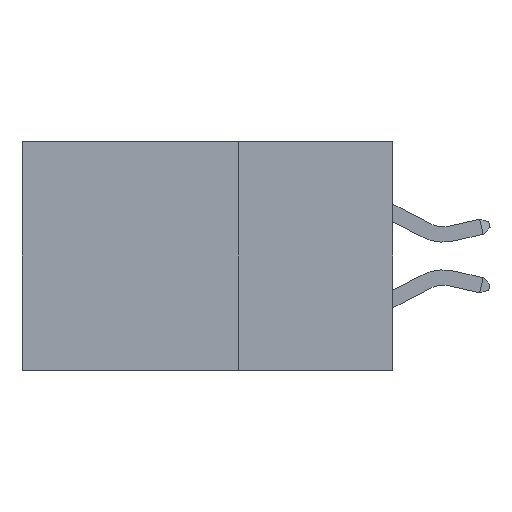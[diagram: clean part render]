
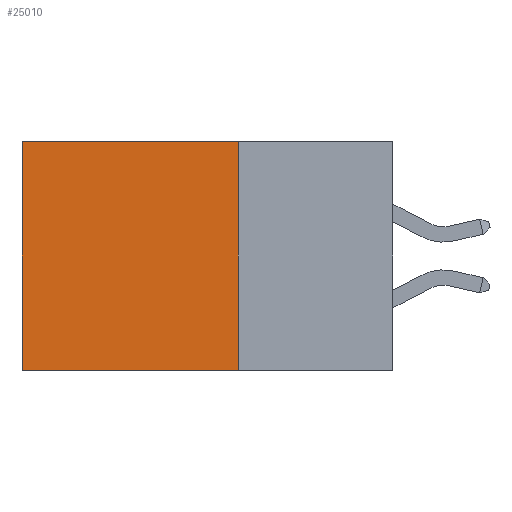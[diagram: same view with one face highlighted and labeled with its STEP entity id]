
A CAD part, left-side view. The second image highlights one B-rep face of the part: STEP entity #25010.
In plain terms, the highlighted planar face has unit normal (-1, 0, 0).
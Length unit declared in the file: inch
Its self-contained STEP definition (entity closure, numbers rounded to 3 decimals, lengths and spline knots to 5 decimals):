
#357 = VECTOR ( 'NONE', #1730, 39.37008 ) ;
#1730 = DIRECTION ( 'NONE',  ( 0., 0., -1. ) ) ;
#2469 = LINE ( 'NONE', #31847, #15809 ) ;
#2660 = DIRECTION ( 'NONE',  ( 0., 1., 0. ) ) ;
#4257 = ORIENTED_EDGE ( 'NONE', *, *, #19604, .F. ) ;
#4283 = CARTESIAN_POINT ( 'NONE',  ( 0.2875, 0.6, -0.37 ) ) ;
#4653 = ORIENTED_EDGE ( 'NONE', *, *, #30574, .T. ) ;
#5959 = CARTESIAN_POINT ( 'NONE',  ( 0.2875, 0.25, -0.37 ) ) ;
#6342 = ORIENTED_EDGE ( 'NONE', *, *, #11516, .T. ) ;
#8146 = DIRECTION ( 'NONE',  ( 0., 0., -1. ) ) ;
#11041 = DIRECTION ( 'NONE',  ( 0., 0., -1. ) ) ;
#11516 = EDGE_CURVE ( 'NONE', #18666, #13287, #2469, .T. ) ;
#12564 = EDGE_LOOP ( 'NONE', ( #4653, #4257, #28218, #6342 ) ) ;
#13007 = PLANE ( 'NONE',  #31144 ) ;
#13287 = VERTEX_POINT ( 'NONE', #31995 ) ;
#13642 = LINE ( 'NONE', #23947, #30734 ) ;
#15809 = VECTOR ( 'NONE', #2660, 39.37008 ) ;
#16402 = CARTESIAN_POINT ( 'NONE',  ( 0.2875, 0.25, 0. ) ) ;
#16793 = DIRECTION ( 'NONE',  ( 0., 1., 0. ) ) ;
#18201 = LINE ( 'NONE', #34817, #357 ) ;
#18666 = VERTEX_POINT ( 'NONE', #16402 ) ;
#18901 = CARTESIAN_POINT ( 'NONE',  ( 0.2875, 0.25, -0.37 ) ) ;
#19369 = VERTEX_POINT ( 'NONE', #18901 ) ;
#19604 = EDGE_CURVE ( 'NONE', #19369, #23159, #30218, .T. ) ;
#22221 = DIRECTION ( 'NONE',  ( 1., 0., 0. ) ) ;
#23159 = VERTEX_POINT ( 'NONE', #4283 ) ;
#23947 = CARTESIAN_POINT ( 'NONE',  ( 0.2875, 0.6, 0. ) ) ;
#24547 = CARTESIAN_POINT ( 'NONE',  ( 0.2875, 0.25, 0. ) ) ;
#25010 = ADVANCED_FACE ( 'NONE', ( #26495 ), #13007, .F. ) ;
#26495 = FACE_OUTER_BOUND ( 'NONE', #12564, .T. ) ;
#28218 = ORIENTED_EDGE ( 'NONE', *, *, #34297, .F. ) ;
#29677 = VECTOR ( 'NONE', #16793, 39.37008 ) ;
#30218 = LINE ( 'NONE', #5959, #29677 ) ;
#30574 = EDGE_CURVE ( 'NONE', #13287, #23159, #13642, .T. ) ;
#30734 = VECTOR ( 'NONE', #8146, 39.37008 ) ;
#31144 = AXIS2_PLACEMENT_3D ( 'NONE', #24547, #22221, #11041 ) ;
#31847 = CARTESIAN_POINT ( 'NONE',  ( 0.2875, 0.25, 0. ) ) ;
#31995 = CARTESIAN_POINT ( 'NONE',  ( 0.2875, 0.6, 0. ) ) ;
#34297 = EDGE_CURVE ( 'NONE', #18666, #19369, #18201, .T. ) ;
#34817 = CARTESIAN_POINT ( 'NONE',  ( 0.2875, 0.25, 0. ) ) ;
